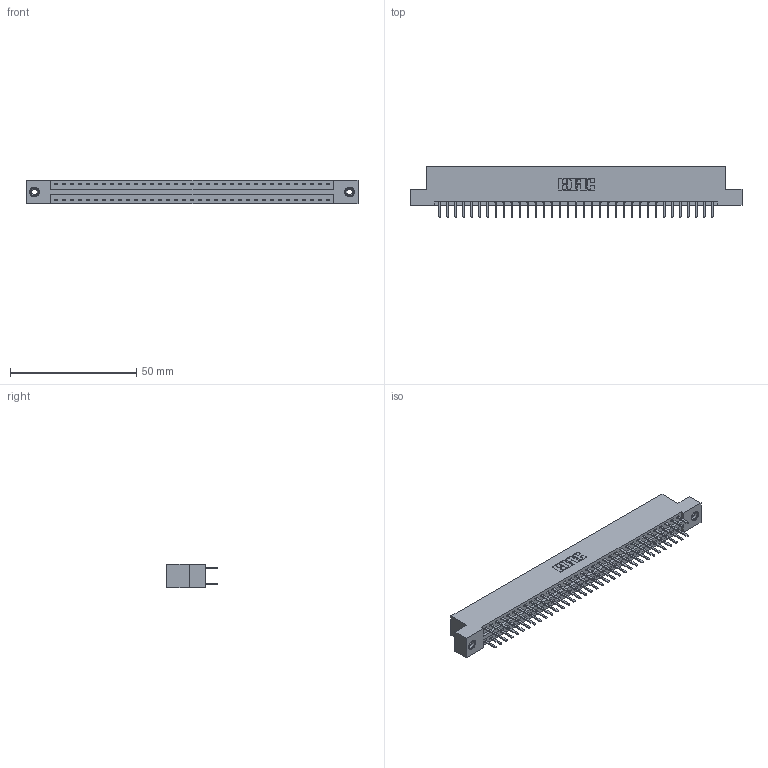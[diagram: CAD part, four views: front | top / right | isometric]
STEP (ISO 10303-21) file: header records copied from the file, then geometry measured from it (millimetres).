
FILE_DESCRIPTION (( 'STEP AP203' ), '1' );
FILE_NAME ('346-070-520-208.STEP', '2018-08-28T22:52:16', ( '' ), ( '' ), 'SwSTEP 2.0', 'SolidWorks 2016', '' );
FILE_SCHEMA (( 'CONFIG_CONTROL_DESIGN' ));
Length unit declared in the file: inch
Products named in the file (4): 346 Part_Flush Mounting Lugs - 0.156 Dia-TI; 345-292-001_345-293-120; 345-250-001_345-250-003-102; 346-070-520-208
Assembly tree (73 placements, depth 2):
  346-070-520-208
    346 Part_Flush Mounting Lugs - 0.156 Dia-TI
    345-292-001_345-293-120  x70
    345-250-001_345-250-003-102  x2
Bounding box: 131.7 x 20.02 x 9.4 mm (x, y, z)
Volume: 12750.6 mm3; surface area: 17364.5 mm2
Topology: 73 solids, 73 shells, 4102 faces, 11875 edges, 7722 vertices
Faces by surface type: plane 2698, cylinder 1388, cone 12, torus 4
Entity records: 25084 total; most frequent: CARTESIAN_POINT 4139, ORIENTED_EDGE 4054, DIRECTION 3713, EDGE_CURVE 2027, VECTOR 1731, LINE 1731, VERTEX_POINT 1344, AXIS2_PLACEMENT_3D 991
